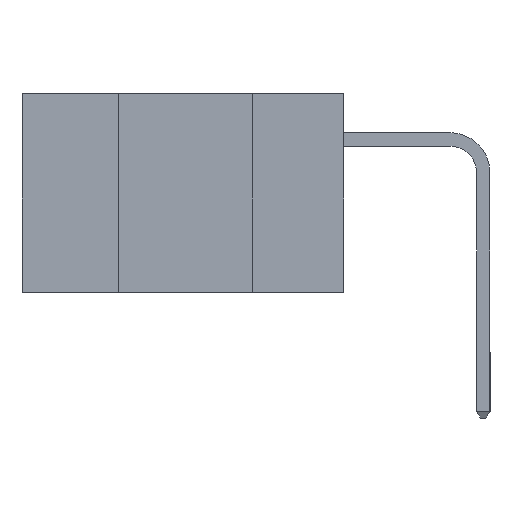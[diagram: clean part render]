
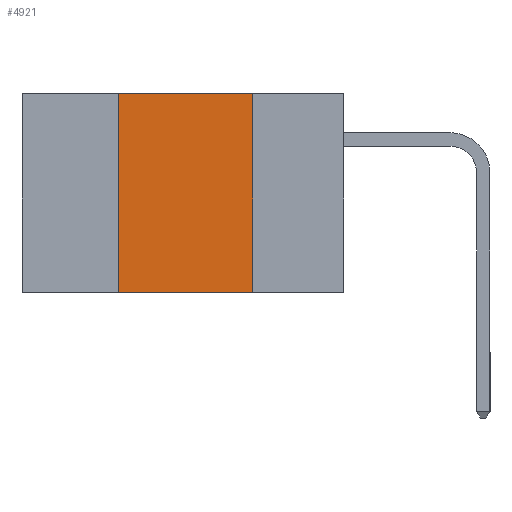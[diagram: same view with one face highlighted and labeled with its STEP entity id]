
A CAD part, left-side view. The second image highlights one B-rep face of the part: STEP entity #4921.
In plain terms, the highlighted planar face has unit normal (-1, 0, 0).
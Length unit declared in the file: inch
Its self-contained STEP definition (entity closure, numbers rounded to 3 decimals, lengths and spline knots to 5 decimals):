
#159 = CARTESIAN_POINT ( 'NONE',  ( 0., 0.6, 0. ) ) ;
#634 = CARTESIAN_POINT ( 'NONE',  ( 0., 0.6, -0.37 ) ) ;
#1222 = VECTOR ( 'NONE', #11101, 39.37008 ) ;
#1353 = EDGE_CURVE ( 'NONE', #5971, #6473, #13240, .T. ) ;
#2212 = ORIENTED_EDGE ( 'NONE', *, *, #7669, .F. ) ;
#2336 = CARTESIAN_POINT ( 'NONE',  ( 0., 0.42, -0.37 ) ) ;
#2368 = LINE ( 'NONE', #10792, #6017 ) ;
#2420 = FACE_OUTER_BOUND ( 'NONE', #12307, .T. ) ;
#2429 = CARTESIAN_POINT ( 'NONE',  ( 0., 0.17, 0. ) ) ;
#2461 = CARTESIAN_POINT ( 'NONE',  ( 0., 0.17, -0.37 ) ) ;
#3128 = VECTOR ( 'NONE', #3203, 39.37008 ) ;
#3203 = DIRECTION ( 'NONE',  ( 0., -1., 0. ) ) ;
#3594 = DIRECTION ( 'NONE',  ( 0., 0., -1. ) ) ;
#3879 = ORIENTED_EDGE ( 'NONE', *, *, #11505, .T. ) ;
#4242 = LINE ( 'NONE', #634, #1222 ) ;
#4921 = ADVANCED_FACE ( 'NONE', ( #2420 ), #14366, .F. ) ;
#5561 = LINE ( 'NONE', #15153, #3128 ) ;
#5971 = VERTEX_POINT ( 'NONE', #2429 ) ;
#6017 = VECTOR ( 'NONE', #15499, 39.37008 ) ;
#6467 = VERTEX_POINT ( 'NONE', #2336 ) ;
#6473 = VERTEX_POINT ( 'NONE', #14209 ) ;
#7669 = EDGE_CURVE ( 'NONE', #12916, #5971, #5561, .T. ) ;
#9725 = DIRECTION ( 'NONE',  ( 1., 0., 0. ) ) ;
#9964 = ORIENTED_EDGE ( 'NONE', *, *, #1353, .F. ) ;
#10290 = VECTOR ( 'NONE', #12072, 39.37008 ) ;
#10310 = ORIENTED_EDGE ( 'NONE', *, *, #14969, .F. ) ;
#10792 = CARTESIAN_POINT ( 'NONE',  ( 0., 0.42, -0.37 ) ) ;
#11101 = DIRECTION ( 'NONE',  ( 0., -1., 0. ) ) ;
#11505 = EDGE_CURVE ( 'NONE', #6467, #6473, #4242, .T. ) ;
#12072 = DIRECTION ( 'NONE',  ( 0., 0., -1. ) ) ;
#12307 = EDGE_LOOP ( 'NONE', ( #9964, #2212, #10310, #3879 ) ) ;
#12916 = VERTEX_POINT ( 'NONE', #14157 ) ;
#13240 = LINE ( 'NONE', #2461, #10290 ) ;
#14157 = CARTESIAN_POINT ( 'NONE',  ( 0., 0.42, 0. ) ) ;
#14165 = AXIS2_PLACEMENT_3D ( 'NONE', #159, #9725, #3594 ) ;
#14209 = CARTESIAN_POINT ( 'NONE',  ( 0., 0.17, -0.37 ) ) ;
#14366 = PLANE ( 'NONE',  #14165 ) ;
#14969 = EDGE_CURVE ( 'NONE', #6467, #12916, #2368, .T. ) ;
#15153 = CARTESIAN_POINT ( 'NONE',  ( 0., 0.6, 0. ) ) ;
#15499 = DIRECTION ( 'NONE',  ( 0., 0., 1. ) ) ;
